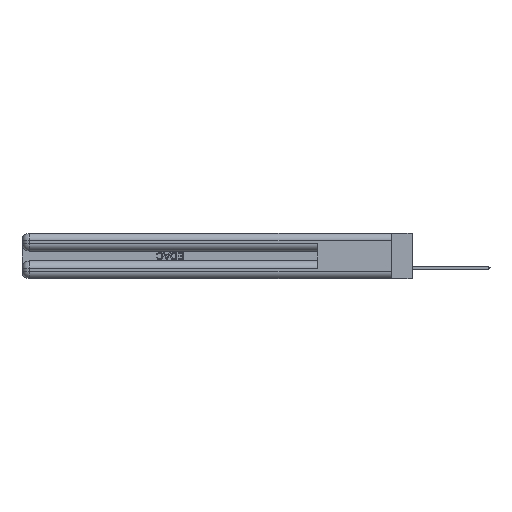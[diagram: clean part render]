
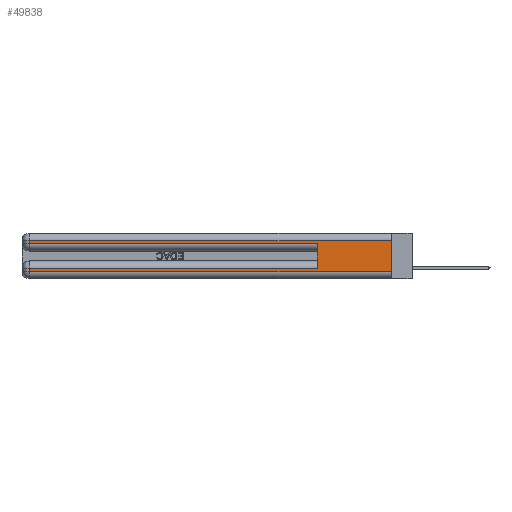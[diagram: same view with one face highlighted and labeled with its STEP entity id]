
A CAD part, left-side view. The second image highlights one B-rep face of the part: STEP entity #49838.
In plain terms, the highlighted planar face has unit normal (-1, 0, 0).
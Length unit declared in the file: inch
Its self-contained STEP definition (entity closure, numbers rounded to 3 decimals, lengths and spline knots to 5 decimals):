
#782 = CARTESIAN_POINT ( 'NONE',  ( 0., 2.94, 0.085 ) ) ;
#1040 = LINE ( 'NONE', #4505, #30126 ) ;
#1544 = VERTEX_POINT ( 'NONE', #2469 ) ;
#2090 = ORIENTED_EDGE ( 'NONE', *, *, #53674, .F. ) ;
#2185 = VECTOR ( 'NONE', #4751, 39.37008 ) ;
#2365 = CARTESIAN_POINT ( 'NONE',  ( 0., 0., 0.37 ) ) ;
#2366 = DIRECTION ( 'NONE',  ( 0., 0., -1. ) ) ;
#2469 = CARTESIAN_POINT ( 'NONE',  ( 0., 0.6, 0.285 ) ) ;
#2876 = ORIENTED_EDGE ( 'NONE', *, *, #24481, .F. ) ;
#2966 = DIRECTION ( 'NONE',  ( 0., 0., -1. ) ) ;
#3724 = LINE ( 'NONE', #15455, #13515 ) ;
#4505 = CARTESIAN_POINT ( 'NONE',  ( 0., 0., 0.285 ) ) ;
#4580 = VERTEX_POINT ( 'NONE', #7764 ) ;
#4677 = AXIS2_PLACEMENT_3D ( 'NONE', #2365, #27305, #2966 ) ;
#4751 = DIRECTION ( 'NONE',  ( 0., 1., 0. ) ) ;
#4982 = EDGE_CURVE ( 'NONE', #13684, #1544, #1040, .T. ) ;
#5090 = ORIENTED_EDGE ( 'NONE', *, *, #4982, .T. ) ;
#7764 = CARTESIAN_POINT ( 'NONE',  ( 0., 2.94, 0.31 ) ) ;
#7765 = VERTEX_POINT ( 'NONE', #48527 ) ;
#8019 = VECTOR ( 'NONE', #52128, 39.37008 ) ;
#8172 = EDGE_CURVE ( 'NONE', #4580, #13684, #37501, .T. ) ;
#8213 = EDGE_CURVE ( 'NONE', #21298, #41174, #46524, .T. ) ;
#8539 = VERTEX_POINT ( 'NONE', #20380 ) ;
#10378 = ORIENTED_EDGE ( 'NONE', *, *, #8172, .T. ) ;
#12551 = EDGE_CURVE ( 'NONE', #41174, #7765, #28578, .T. ) ;
#13421 = CARTESIAN_POINT ( 'NONE',  ( 0., 0., 0.31 ) ) ;
#13515 = VECTOR ( 'NONE', #19651, 39.37008 ) ;
#13684 = VERTEX_POINT ( 'NONE', #24515 ) ;
#15455 = CARTESIAN_POINT ( 'NONE',  ( 0., 0., 0.06 ) ) ;
#16260 = LINE ( 'NONE', #52208, #53558 ) ;
#16378 = LINE ( 'NONE', #32441, #41248 ) ;
#18824 = ORIENTED_EDGE ( 'NONE', *, *, #8213, .T. ) ;
#18864 = CARTESIAN_POINT ( 'NONE',  ( 0., 2.94, 0.37 ) ) ;
#19651 = DIRECTION ( 'NONE',  ( 0., -1., 0. ) ) ;
#19981 = LINE ( 'NONE', #13421, #2185 ) ;
#20380 = CARTESIAN_POINT ( 'NONE',  ( 0., 0., 0.06 ) ) ;
#21298 = VERTEX_POINT ( 'NONE', #31288 ) ;
#24481 = EDGE_CURVE ( 'NONE', #37684, #8539, #16260, .T. ) ;
#24515 = CARTESIAN_POINT ( 'NONE',  ( 0., 2.94, 0.285 ) ) ;
#25071 = ORIENTED_EDGE ( 'NONE', *, *, #27766, .T. ) ;
#26251 = VECTOR ( 'NONE', #47898, 39.37008 ) ;
#26493 = VECTOR ( 'NONE', #2366, 39.37008 ) ;
#27305 = DIRECTION ( 'NONE',  ( 1., 0., 0. ) ) ;
#27766 = EDGE_CURVE ( 'NONE', #7765, #8539, #3724, .T. ) ;
#28578 = LINE ( 'NONE', #18864, #26493 ) ;
#30126 = VECTOR ( 'NONE', #38175, 39.37008 ) ;
#31017 = DIRECTION ( 'NONE',  ( 0., 0., -1. ) ) ;
#31288 = CARTESIAN_POINT ( 'NONE',  ( 0., 0.6, 0.085 ) ) ;
#32441 = CARTESIAN_POINT ( 'NONE',  ( 0., 0.6, 0.145 ) ) ;
#35365 = FACE_OUTER_BOUND ( 'NONE', #51865, .T. ) ;
#37501 = LINE ( 'NONE', #40338, #26251 ) ;
#37684 = VERTEX_POINT ( 'NONE', #40025 ) ;
#38175 = DIRECTION ( 'NONE',  ( 0., -1., 0. ) ) ;
#40025 = CARTESIAN_POINT ( 'NONE',  ( 0., 0., 0.31 ) ) ;
#40338 = CARTESIAN_POINT ( 'NONE',  ( 0., 2.94, 0.37 ) ) ;
#41174 = VERTEX_POINT ( 'NONE', #782 ) ;
#41248 = VECTOR ( 'NONE', #53035, 39.37008 ) ;
#41388 = ORIENTED_EDGE ( 'NONE', *, *, #49588, .T. ) ;
#46524 = LINE ( 'NONE', #48505, #8019 ) ;
#47898 = DIRECTION ( 'NONE',  ( 0., 0., -1. ) ) ;
#48291 = PLANE ( 'NONE',  #4677 ) ;
#48505 = CARTESIAN_POINT ( 'NONE',  ( 0., 0., 0.085 ) ) ;
#48527 = CARTESIAN_POINT ( 'NONE',  ( 0., 2.94, 0.06 ) ) ;
#49588 = EDGE_CURVE ( 'NONE', #37684, #4580, #19981, .T. ) ;
#49838 = ADVANCED_FACE ( 'NONE', ( #35365 ), #48291, .F. ) ;
#51865 = EDGE_LOOP ( 'NONE', ( #2876, #41388, #10378, #5090, #2090, #18824, #53180, #25071 ) ) ;
#52128 = DIRECTION ( 'NONE',  ( 0., 1., 0. ) ) ;
#52208 = CARTESIAN_POINT ( 'NONE',  ( 0., 0., 0.37 ) ) ;
#53035 = DIRECTION ( 'NONE',  ( 0., 0., 1. ) ) ;
#53180 = ORIENTED_EDGE ( 'NONE', *, *, #12551, .T. ) ;
#53558 = VECTOR ( 'NONE', #31017, 39.37008 ) ;
#53674 = EDGE_CURVE ( 'NONE', #21298, #1544, #16378, .T. ) ;
